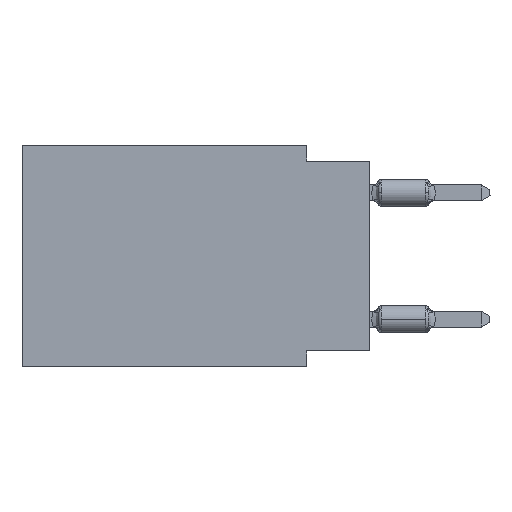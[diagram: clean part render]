
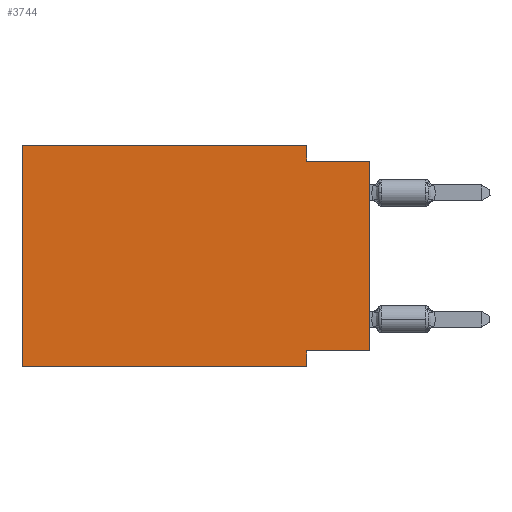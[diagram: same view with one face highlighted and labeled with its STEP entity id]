
A CAD part, left-side view. The second image highlights one B-rep face of the part: STEP entity #3744.
In plain terms, the highlighted planar face has unit normal (-1, 0, 0).
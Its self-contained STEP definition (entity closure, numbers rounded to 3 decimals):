
#7 = DIRECTION ( 'NONE',  ( 0., 0., 1. ) ) ;
#843 = CARTESIAN_POINT ( 'NONE',  ( 0., 2.54, 0. ) ) ;
#1070 = EDGE_CURVE ( 'NONE', #18687, #6645, #14606, .T. ) ;
#1881 = CARTESIAN_POINT ( 'NONE',  ( 0., 2.54, -8.89 ) ) ;
#3005 = CARTESIAN_POINT ( 'NONE',  ( 0., 13.97, 0. ) ) ;
#3548 = CARTESIAN_POINT ( 'NONE',  ( 0., 0., 0. ) ) ;
#3646 = CARTESIAN_POINT ( 'NONE',  ( 0., 0., -8.255 ) ) ;
#3744 = ADVANCED_FACE ( 'NONE', ( #20530 ), #13417, .F. ) ;
#3791 = VECTOR ( 'NONE', #13458, 1000. ) ;
#4396 = VECTOR ( 'NONE', #6170, 1000. ) ;
#5081 = ORIENTED_EDGE ( 'NONE', *, *, #14283, .T. ) ;
#6118 = ORIENTED_EDGE ( 'NONE', *, *, #14476, .F. ) ;
#6170 = DIRECTION ( 'NONE',  ( 0., 0., 1. ) ) ;
#6337 = VECTOR ( 'NONE', #17825, 1000. ) ;
#6572 = ORIENTED_EDGE ( 'NONE', *, *, #1070, .F. ) ;
#6645 = VERTEX_POINT ( 'NONE', #1881 ) ;
#6785 = CARTESIAN_POINT ( 'NONE',  ( 0., 13.97, -8.89 ) ) ;
#6871 = DIRECTION ( 'NONE',  ( 0., 1., 0. ) ) ;
#6909 = CARTESIAN_POINT ( 'NONE',  ( 0., 2.54, -8.255 ) ) ;
#7082 = VECTOR ( 'NONE', #6871, 1000. ) ;
#8691 = VECTOR ( 'NONE', #12876, 1000. ) ;
#8899 = CARTESIAN_POINT ( 'NONE',  ( 0., 2.54, 0. ) ) ;
#9052 = ORIENTED_EDGE ( 'NONE', *, *, #19383, .F. ) ;
#9197 = EDGE_CURVE ( 'NONE', #11470, #13272, #15046, .T. ) ;
#9297 = LINE ( 'NONE', #16457, #6337 ) ;
#9635 = LINE ( 'NONE', #9739, #17816 ) ;
#9739 = CARTESIAN_POINT ( 'NONE',  ( 0., 0., -0.635 ) ) ;
#10282 = CARTESIAN_POINT ( 'NONE',  ( 0., 13.97, 0. ) ) ;
#10542 = LINE ( 'NONE', #3646, #7082 ) ;
#11298 = LINE ( 'NONE', #843, #3791 ) ;
#11386 = EDGE_CURVE ( 'NONE', #13272, #12449, #16927, .T. ) ;
#11470 = VERTEX_POINT ( 'NONE', #6785 ) ;
#12365 = AXIS2_PLACEMENT_3D ( 'NONE', #10282, #20415, #17317 ) ;
#12378 = VERTEX_POINT ( 'NONE', #16173 ) ;
#12449 = VERTEX_POINT ( 'NONE', #8899 ) ;
#12743 = CARTESIAN_POINT ( 'NONE',  ( 0., 13.97, 0. ) ) ;
#12876 = DIRECTION ( 'NONE',  ( 0., 0., -1. ) ) ;
#12974 = ORIENTED_EDGE ( 'NONE', *, *, #22196, .T. ) ;
#13272 = VERTEX_POINT ( 'NONE', #12743 ) ;
#13417 = PLANE ( 'NONE',  #12365 ) ;
#13458 = DIRECTION ( 'NONE',  ( 0., 0., -1. ) ) ;
#14283 = EDGE_CURVE ( 'NONE', #11470, #6645, #9297, .T. ) ;
#14464 = EDGE_CURVE ( 'NONE', #12449, #19328, #11298, .T. ) ;
#14476 = EDGE_CURVE ( 'NONE', #12378, #18687, #10542, .T. ) ;
#14606 = LINE ( 'NONE', #19654, #8691 ) ;
#15046 = LINE ( 'NONE', #20218, #4396 ) ;
#16173 = CARTESIAN_POINT ( 'NONE',  ( 0., 0., -8.255 ) ) ;
#16457 = CARTESIAN_POINT ( 'NONE',  ( 0., 13.97, -8.89 ) ) ;
#16748 = VECTOR ( 'NONE', #7, 1000. ) ;
#16876 = ORIENTED_EDGE ( 'NONE', *, *, #14464, .F. ) ;
#16927 = LINE ( 'NONE', #3005, #18814 ) ;
#17102 = DIRECTION ( 'NONE',  ( 0., -1., 0. ) ) ;
#17152 = DIRECTION ( 'NONE',  ( 0., -1., 0. ) ) ;
#17214 = ORIENTED_EDGE ( 'NONE', *, *, #11386, .F. ) ;
#17317 = DIRECTION ( 'NONE',  ( 0., 0., -1. ) ) ;
#17494 = VERTEX_POINT ( 'NONE', #19999 ) ;
#17816 = VECTOR ( 'NONE', #17102, 1000. ) ;
#17825 = DIRECTION ( 'NONE',  ( 0., -1., 0. ) ) ;
#18687 = VERTEX_POINT ( 'NONE', #6909 ) ;
#18814 = VECTOR ( 'NONE', #17152, 1000. ) ;
#18835 = CARTESIAN_POINT ( 'NONE',  ( 0., 2.54, -0.635 ) ) ;
#19328 = VERTEX_POINT ( 'NONE', #18835 ) ;
#19383 = EDGE_CURVE ( 'NONE', #19328, #17494, #9635, .T. ) ;
#19654 = CARTESIAN_POINT ( 'NONE',  ( 0., 2.54, -8.89 ) ) ;
#19774 = LINE ( 'NONE', #3548, #16748 ) ;
#19999 = CARTESIAN_POINT ( 'NONE',  ( 0., 0., -0.635 ) ) ;
#20218 = CARTESIAN_POINT ( 'NONE',  ( 0., 13.97, 0. ) ) ;
#20415 = DIRECTION ( 'NONE',  ( 1., 0., 0. ) ) ;
#20530 = FACE_OUTER_BOUND ( 'NONE', #21333, .T. ) ;
#20721 = ORIENTED_EDGE ( 'NONE', *, *, #9197, .F. ) ;
#21333 = EDGE_LOOP ( 'NONE', ( #12974, #9052, #16876, #17214, #20721, #5081, #6572, #6118 ) ) ;
#22196 = EDGE_CURVE ( 'NONE', #12378, #17494, #19774, .T. ) ;
